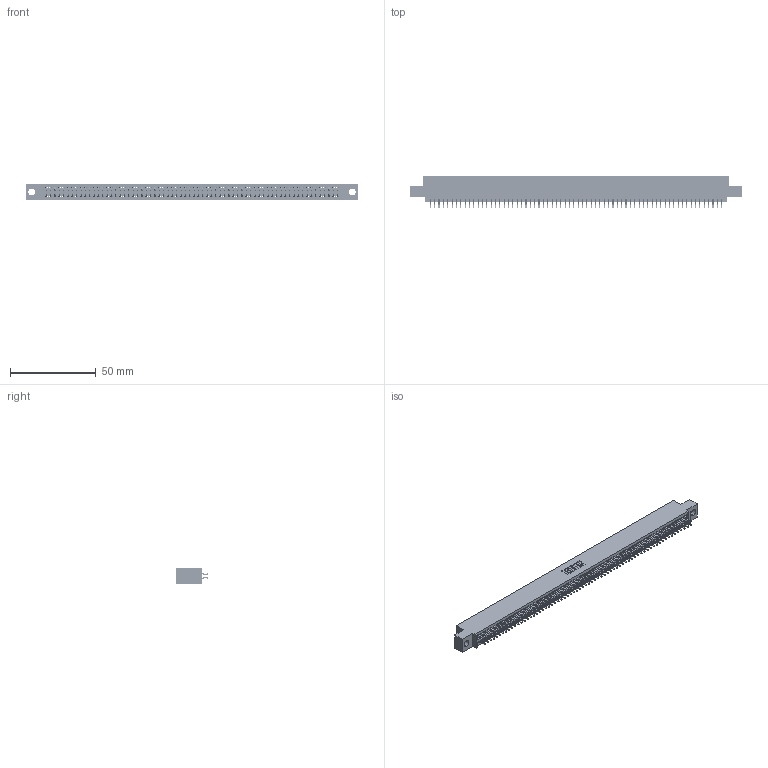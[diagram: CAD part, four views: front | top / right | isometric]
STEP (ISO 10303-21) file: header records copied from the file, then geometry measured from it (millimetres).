
FILE_DESCRIPTION (( 'STEP AP203' ), '1' );
FILE_NAME ('395-136-556-504.STEP', '2018-12-05T10:40:51', ( '' ), ( '' ), 'SwSTEP 2.0', 'SolidWorks 2016', '' );
FILE_SCHEMA (( 'CONFIG_CONTROL_DESIGN' ));
Length unit declared in the file: inch
Products named in the file (3): 345-292-001_556 Tail; 345 Part_0.110 Offset - 0.156 Dia-TH; 395-136-556-504
Assembly tree (137 placements, depth 2):
  395-136-556-504
    345 Part_0.110 Offset - 0.156 Dia-TH
    345-292-001_556 Tail  x136
Bounding box: 193.93 x 19.24 x 9.4 mm (x, y, z)
Volume: 18913.2 mm3; surface area: 28249.4 mm2
Topology: 137 solids, 137 shells, 7746 faces, 23065 edges, 15194 vertices
Faces by surface type: plane 5116, cylinder 2630
Entity records: 50209 total; most frequent: CARTESIAN_POINT 8408, ORIENTED_EDGE 8330, DIRECTION 7369, EDGE_CURVE 4165, VECTOR 3753, LINE 3753, VERTEX_POINT 2774, AXIS2_PLACEMENT_3D 1808
